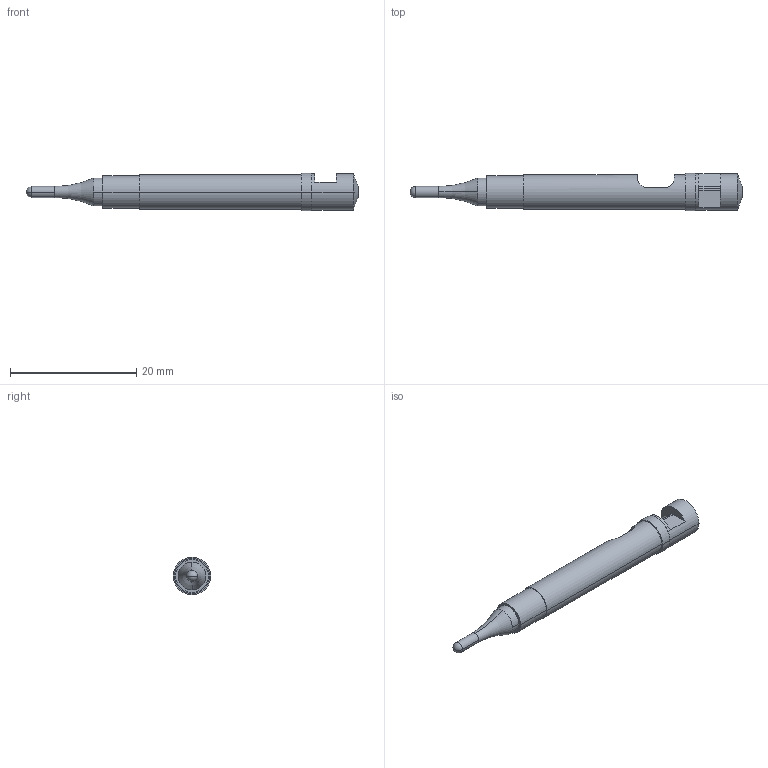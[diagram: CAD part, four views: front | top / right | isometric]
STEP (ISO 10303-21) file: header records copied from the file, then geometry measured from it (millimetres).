
FILE_DESCRIPTION (( 'STEP AP214' ), '1' );
FILE_NAME ('Firing Pin.step', '2014-07-30T19:45:47', ( 'WarFairy' ), ( '' ), 'SwSTEP 2.0', 'SolidWorks 2013', '' );
FILE_SCHEMA (( 'AUTOMOTIVE_DESIGN' ));
Length unit declared in the file: millimetre
Products named in the file (1): Firing Pin
Bounding box: 52.57 x 5.94 x 5.94 mm (x, y, z)
Volume: 961.8 mm3; surface area: 834.8 mm2
Topology: 1 solids, 1 shells, 34 faces, 85 edges, 55 vertices
Faces by surface type: cylinder 16, plane 12, cone 2, torus 2, sphere 2
Entity records: 1081 total; most frequent: CARTESIAN_POINT 217, DIRECTION 193, ORIENTED_EDGE 162, AXIS2_PLACEMENT_3D 81, EDGE_CURVE 81, VERTEX_POINT 53, CIRCLE 46, EDGE_LOOP 38
